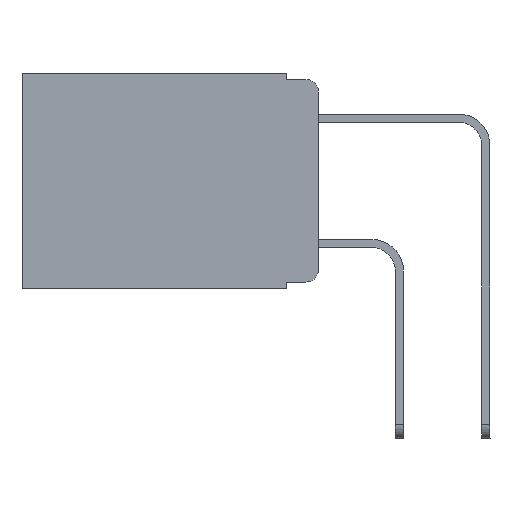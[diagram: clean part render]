
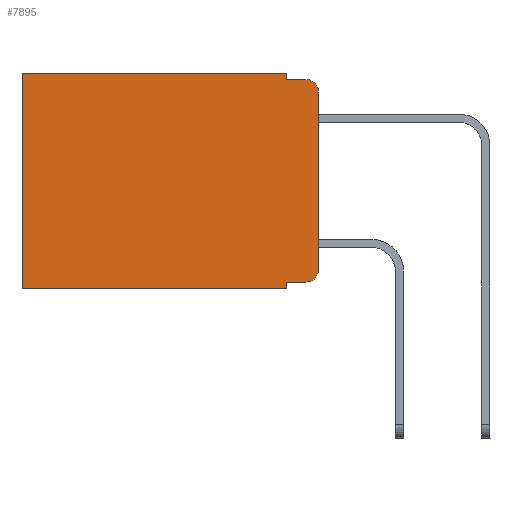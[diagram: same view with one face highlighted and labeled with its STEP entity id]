
A CAD part, left-side view. The second image highlights one B-rep face of the part: STEP entity #7895.
In plain terms, the highlighted planar face has unit normal (-1, 0, 0).
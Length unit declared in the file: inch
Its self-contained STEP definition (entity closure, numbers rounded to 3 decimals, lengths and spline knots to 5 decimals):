
#184 = VECTOR ( 'NONE', #899, 39.37008 ) ;
#266 = PLANE ( 'NONE',  #2360 ) ;
#341 = DIRECTION ( 'NONE',  ( 0., 1., 0. ) ) ;
#479 = VERTEX_POINT ( 'NONE', #5285 ) ;
#783 = DIRECTION ( 'NONE',  ( 0., -1., 0. ) ) ;
#882 = DIRECTION ( 'NONE',  ( -1., 0., 0. ) ) ;
#899 = DIRECTION ( 'NONE',  ( 0., 0., -1. ) ) ;
#1054 = VERTEX_POINT ( 'NONE', #8668 ) ;
#1221 = LINE ( 'NONE', #10388, #9662 ) ;
#1365 = DIRECTION ( 'NONE',  ( 1., 0., 0. ) ) ;
#1692 = ORIENTED_EDGE ( 'NONE', *, *, #5990, .T. ) ;
#1707 = LINE ( 'NONE', #9182, #8200 ) ;
#1722 = VECTOR ( 'NONE', #3099, 39.37008 ) ;
#2042 = LINE ( 'NONE', #5799, #1722 ) ;
#2153 = CARTESIAN_POINT ( 'NONE',  ( 0.298, 0.051, -0.343 ) ) ;
#2217 = VECTOR ( 'NONE', #2727, 39.37008 ) ;
#2360 = AXIS2_PLACEMENT_3D ( 'NONE', #8875, #1365, #7498 ) ;
#2371 = ORIENTED_EDGE ( 'NONE', *, *, #7733, .F. ) ;
#2727 = DIRECTION ( 'NONE',  ( 0., 0., -1. ) ) ;
#2813 = VERTEX_POINT ( 'NONE', #4237 ) ;
#2828 = VECTOR ( 'NONE', #341, 39.37008 ) ;
#2951 = FACE_OUTER_BOUND ( 'NONE', #6147, .T. ) ;
#2969 = ORIENTED_EDGE ( 'NONE', *, *, #6038, .F. ) ;
#3099 = DIRECTION ( 'NONE',  ( 0., 0., -1. ) ) ;
#3358 = CARTESIAN_POINT ( 'NONE',  ( 0.298, 0., -0.03 ) ) ;
#3435 = ORIENTED_EDGE ( 'NONE', *, *, #5750, .F. ) ;
#3589 = VERTEX_POINT ( 'NONE', #3827 ) ;
#3827 = CARTESIAN_POINT ( 'NONE',  ( 0.298, 0., -0.313 ) ) ;
#3957 = VERTEX_POINT ( 'NONE', #3358 ) ;
#4190 = LINE ( 'NONE', #5267, #2828 ) ;
#4237 = CARTESIAN_POINT ( 'NONE',  ( 0.298, 0.02, -0.01 ) ) ;
#4512 = LINE ( 'NONE', #8419, #2217 ) ;
#4692 = DIRECTION ( 'NONE',  ( -1., 0., 0. ) ) ;
#4723 = DIRECTION ( 'NONE',  ( 0., -1., 0. ) ) ;
#4785 = VERTEX_POINT ( 'NONE', #9718 ) ;
#4917 = LINE ( 'NONE', #9951, #5426 ) ;
#4946 = DIRECTION ( 'NONE',  ( 0., 0., -1. ) ) ;
#5004 = CARTESIAN_POINT ( 'NONE',  ( 0.298, 0., -0.343 ) ) ;
#5185 = VERTEX_POINT ( 'NONE', #2153 ) ;
#5267 = CARTESIAN_POINT ( 'NONE',  ( 0.298, 0., 0. ) ) ;
#5285 = CARTESIAN_POINT ( 'NONE',  ( 0.298, 0.473, 0. ) ) ;
#5426 = VECTOR ( 'NONE', #4946, 39.37008 ) ;
#5524 = AXIS2_PLACEMENT_3D ( 'NONE', #6404, #882, #7161 ) ;
#5750 = EDGE_CURVE ( 'NONE', #3957, #3589, #4512, .T. ) ;
#5766 = EDGE_CURVE ( 'NONE', #3957, #2813, #10046, .T. ) ;
#5784 = EDGE_CURVE ( 'NONE', #6390, #2813, #1221, .T. ) ;
#5799 = CARTESIAN_POINT ( 'NONE',  ( 0.298, 0.051, 0. ) ) ;
#5906 = EDGE_CURVE ( 'NONE', #8845, #6390, #7665, .T. ) ;
#5914 = ORIENTED_EDGE ( 'NONE', *, *, #7186, .T. ) ;
#5990 = EDGE_CURVE ( 'NONE', #479, #8456, #4917, .T. ) ;
#6034 = CIRCLE ( 'NONE', #5524, 0.02 ) ;
#6038 = EDGE_CURVE ( 'NONE', #4785, #5185, #2042, .T. ) ;
#6147 = EDGE_LOOP ( 'NONE', ( #3435, #9736, #7604, #9544, #5914, #1692, #2371, #2969, #9908, #9520 ) ) ;
#6390 = VERTEX_POINT ( 'NONE', #8227 ) ;
#6404 = CARTESIAN_POINT ( 'NONE',  ( 0.298, 0.02, -0.313 ) ) ;
#6813 = EDGE_CURVE ( 'NONE', #4785, #1054, #1707, .T. ) ;
#6912 = EDGE_CURVE ( 'NONE', #1054, #3589, #6034, .T. ) ;
#7161 = DIRECTION ( 'NONE',  ( 0., 0., -1. ) ) ;
#7186 = EDGE_CURVE ( 'NONE', #8845, #479, #4190, .T. ) ;
#7498 = DIRECTION ( 'NONE',  ( 0., 0., -1. ) ) ;
#7604 = ORIENTED_EDGE ( 'NONE', *, *, #5784, .F. ) ;
#7665 = LINE ( 'NONE', #9255, #184 ) ;
#7733 = EDGE_CURVE ( 'NONE', #5185, #8456, #8515, .T. ) ;
#7809 = CARTESIAN_POINT ( 'NONE',  ( 0.298, 0.473, -0.343 ) ) ;
#7829 = AXIS2_PLACEMENT_3D ( 'NONE', #9136, #4692, #9763 ) ;
#7895 = ADVANCED_FACE ( 'NONE', ( #2951 ), #266, .F. ) ;
#8200 = VECTOR ( 'NONE', #783, 39.37008 ) ;
#8227 = CARTESIAN_POINT ( 'NONE',  ( 0.298, 0.051, -0.01 ) ) ;
#8296 = VECTOR ( 'NONE', #9373, 39.37008 ) ;
#8419 = CARTESIAN_POINT ( 'NONE',  ( 0.298, 0., 0. ) ) ;
#8456 = VERTEX_POINT ( 'NONE', #7809 ) ;
#8515 = LINE ( 'NONE', #5004, #8296 ) ;
#8668 = CARTESIAN_POINT ( 'NONE',  ( 0.298, 0.02, -0.333 ) ) ;
#8845 = VERTEX_POINT ( 'NONE', #10034 ) ;
#8875 = CARTESIAN_POINT ( 'NONE',  ( 0.298, 0., 0. ) ) ;
#9136 = CARTESIAN_POINT ( 'NONE',  ( 0.298, 0.02, -0.03 ) ) ;
#9182 = CARTESIAN_POINT ( 'NONE',  ( 0.298, 0.051, -0.333 ) ) ;
#9255 = CARTESIAN_POINT ( 'NONE',  ( 0.298, 0.051, 0. ) ) ;
#9373 = DIRECTION ( 'NONE',  ( 0., 1., 0. ) ) ;
#9520 = ORIENTED_EDGE ( 'NONE', *, *, #6912, .T. ) ;
#9544 = ORIENTED_EDGE ( 'NONE', *, *, #5906, .F. ) ;
#9662 = VECTOR ( 'NONE', #4723, 39.37008 ) ;
#9718 = CARTESIAN_POINT ( 'NONE',  ( 0.298, 0.051, -0.333 ) ) ;
#9736 = ORIENTED_EDGE ( 'NONE', *, *, #5766, .T. ) ;
#9763 = DIRECTION ( 'NONE',  ( 0., 0., -1. ) ) ;
#9908 = ORIENTED_EDGE ( 'NONE', *, *, #6813, .T. ) ;
#9951 = CARTESIAN_POINT ( 'NONE',  ( 0.298, 0.473, 0. ) ) ;
#10034 = CARTESIAN_POINT ( 'NONE',  ( 0.298, 0.051, 0. ) ) ;
#10046 = CIRCLE ( 'NONE', #7829, 0.02 ) ;
#10388 = CARTESIAN_POINT ( 'NONE',  ( 0.298, 0.051, -0.01 ) ) ;
